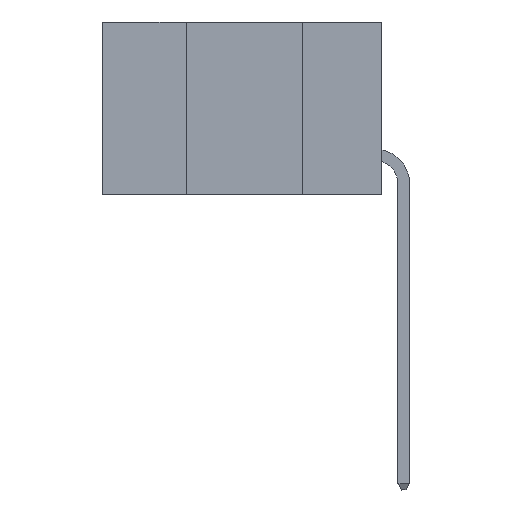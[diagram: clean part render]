
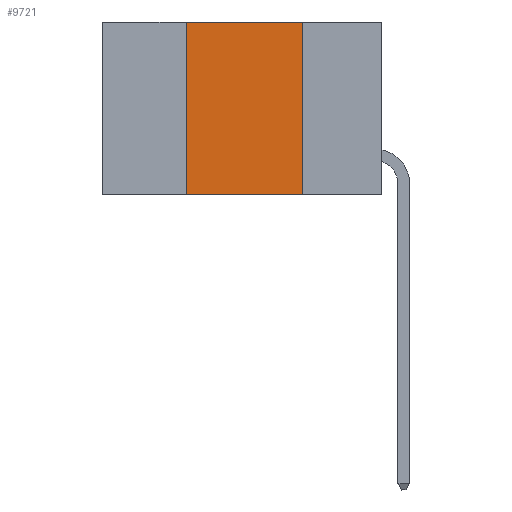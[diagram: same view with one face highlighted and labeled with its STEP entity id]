
A CAD part, left-side view. The second image highlights one B-rep face of the part: STEP entity #9721.
In plain terms, the highlighted planar face has unit normal (-1, 0, 0).
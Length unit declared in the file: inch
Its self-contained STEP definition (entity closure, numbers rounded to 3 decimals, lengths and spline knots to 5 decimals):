
#537 = VERTEX_POINT ( 'NONE', #16849 ) ;
#669 = DIRECTION ( 'NONE',  ( 0., 0., 1. ) ) ;
#895 = LINE ( 'NONE', #6969, #22231 ) ;
#2106 = CARTESIAN_POINT ( 'NONE',  ( 0., 0.17, 0. ) ) ;
#2605 = EDGE_CURVE ( 'NONE', #537, #12964, #20684, .T. ) ;
#3135 = CARTESIAN_POINT ( 'NONE',  ( 0., 0.42, 0. ) ) ;
#4728 = ORIENTED_EDGE ( 'NONE', *, *, #23811, .F. ) ;
#5835 = DIRECTION ( 'NONE',  ( 1., 0., 0. ) ) ;
#5942 = CARTESIAN_POINT ( 'NONE',  ( 0., 0.17, -0.37 ) ) ;
#6603 = VECTOR ( 'NONE', #10169, 39.37008 ) ;
#6969 = CARTESIAN_POINT ( 'NONE',  ( 0., 0.6, -0.37 ) ) ;
#8209 = FACE_OUTER_BOUND ( 'NONE', #22266, .T. ) ;
#8388 = CARTESIAN_POINT ( 'NONE',  ( 0., 0.17, 0. ) ) ;
#9518 = LINE ( 'NONE', #3135, #14176 ) ;
#9721 = ADVANCED_FACE ( 'NONE', ( #8209 ), #24940, .F. ) ;
#9741 = CARTESIAN_POINT ( 'NONE',  ( 0., 0.42, -0.37 ) ) ;
#10169 = DIRECTION ( 'NONE',  ( 0., -1., 0. ) ) ;
#10730 = EDGE_CURVE ( 'NONE', #25033, #14429, #895, .T. ) ;
#11007 = DIRECTION ( 'NONE',  ( 0., -1., 0. ) ) ;
#12964 = VERTEX_POINT ( 'NONE', #2106 ) ;
#14176 = VECTOR ( 'NONE', #669, 39.37008 ) ;
#14429 = VERTEX_POINT ( 'NONE', #5942 ) ;
#14710 = DIRECTION ( 'NONE',  ( 0., 0., -1. ) ) ;
#15537 = VECTOR ( 'NONE', #20712, 39.37008 ) ;
#16849 = CARTESIAN_POINT ( 'NONE',  ( 0., 0.42, 0. ) ) ;
#19548 = AXIS2_PLACEMENT_3D ( 'NONE', #25071, #5835, #14710 ) ;
#20438 = LINE ( 'NONE', #8388, #15537 ) ;
#20684 = LINE ( 'NONE', #24570, #6603 ) ;
#20712 = DIRECTION ( 'NONE',  ( 0., 0., -1. ) ) ;
#22231 = VECTOR ( 'NONE', #11007, 39.37008 ) ;
#22266 = EDGE_LOOP ( 'NONE', ( #4728, #25242, #22905, #25392 ) ) ;
#22402 = EDGE_CURVE ( 'NONE', #25033, #537, #9518, .T. ) ;
#22905 = ORIENTED_EDGE ( 'NONE', *, *, #22402, .F. ) ;
#23811 = EDGE_CURVE ( 'NONE', #12964, #14429, #20438, .T. ) ;
#24570 = CARTESIAN_POINT ( 'NONE',  ( 0., 0.6, 0. ) ) ;
#24940 = PLANE ( 'NONE',  #19548 ) ;
#25033 = VERTEX_POINT ( 'NONE', #9741 ) ;
#25071 = CARTESIAN_POINT ( 'NONE',  ( 0., 0.6, 0. ) ) ;
#25242 = ORIENTED_EDGE ( 'NONE', *, *, #2605, .F. ) ;
#25392 = ORIENTED_EDGE ( 'NONE', *, *, #10730, .T. ) ;
